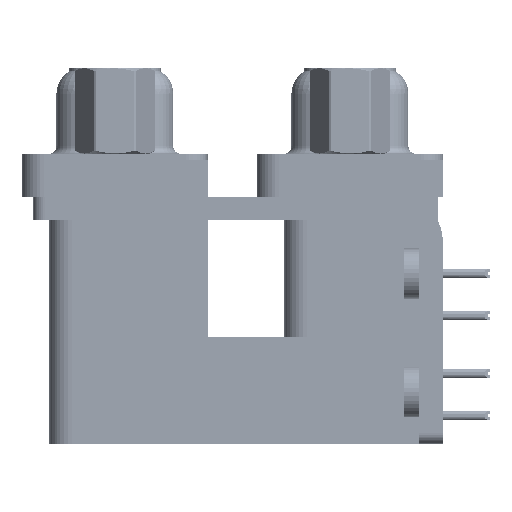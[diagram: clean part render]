
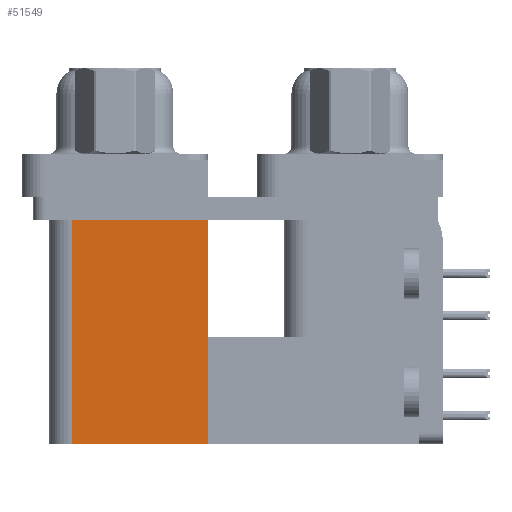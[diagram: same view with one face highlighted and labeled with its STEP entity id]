
A CAD part, left-side view. The second image highlights one B-rep face of the part: STEP entity #51549.
In plain terms, the highlighted planar face has unit normal (-1, 0, 0).
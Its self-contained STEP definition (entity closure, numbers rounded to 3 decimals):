
#265 = DIRECTION ( 'NONE',  ( 0., 0., 1. ) ) ;
#1208 = LINE ( 'NONE', #51632, #34394 ) ;
#1245 = VERTEX_POINT ( 'NONE', #5433 ) ;
#2728 = DIRECTION ( 'NONE',  ( 0., 1., 0. ) ) ;
#2841 = VECTOR ( 'NONE', #73169, 1000. ) ;
#5433 = CARTESIAN_POINT ( 'NONE',  ( 3.79, 18.8, -19.2 ) ) ;
#5642 = VERTEX_POINT ( 'NONE', #30023 ) ;
#8924 = LINE ( 'NONE', #34158, #12694 ) ;
#11295 = EDGE_CURVE ( 'NONE', #75592, #13830, #1208, .T. ) ;
#11579 = PLANE ( 'NONE',  #75513 ) ;
#11611 = ORIENTED_EDGE ( 'NONE', *, *, #14399, .F. ) ;
#12694 = VECTOR ( 'NONE', #2728, 1000. ) ;
#13830 = VERTEX_POINT ( 'NONE', #38008 ) ;
#14399 = EDGE_CURVE ( 'NONE', #75592, #1245, #8924, .T. ) ;
#16009 = CARTESIAN_POINT ( 'NONE',  ( 3.79, 9.6, -19.2 ) ) ;
#23456 = EDGE_CURVE ( 'NONE', #13830, #5642, #47955, .T. ) ;
#28058 = EDGE_CURVE ( 'NONE', #1245, #5642, #62277, .T. ) ;
#29595 = EDGE_LOOP ( 'NONE', ( #60127, #52604, #11611, #73415 ) ) ;
#30023 = CARTESIAN_POINT ( 'NONE',  ( 3.79, 18.8, -2.5 ) ) ;
#34158 = CARTESIAN_POINT ( 'NONE',  ( 3.79, 9.6, -19.2 ) ) ;
#34394 = VECTOR ( 'NONE', #64431, 1000. ) ;
#36811 = CARTESIAN_POINT ( 'NONE',  ( 3.79, 9.6, -19.2 ) ) ;
#38008 = CARTESIAN_POINT ( 'NONE',  ( 3.79, 9.6, -2.5 ) ) ;
#40959 = CARTESIAN_POINT ( 'NONE',  ( 3.79, 9.6, -2.5 ) ) ;
#43399 = DIRECTION ( 'NONE',  ( 0., 0., -1. ) ) ;
#47340 = VECTOR ( 'NONE', #265, 1000. ) ;
#47955 = LINE ( 'NONE', #40959, #2841 ) ;
#51549 = ADVANCED_FACE ( 'NONE', ( #68217 ), #11579, .F. ) ;
#51632 = CARTESIAN_POINT ( 'NONE',  ( 3.79, 9.6, -19.2 ) ) ;
#52604 = ORIENTED_EDGE ( 'NONE', *, *, #28058, .F. ) ;
#60127 = ORIENTED_EDGE ( 'NONE', *, *, #23456, .T. ) ;
#62277 = LINE ( 'NONE', #80488, #47340 ) ;
#64431 = DIRECTION ( 'NONE',  ( 0., 0., 1. ) ) ;
#68217 = FACE_OUTER_BOUND ( 'NONE', #29595, .T. ) ;
#73169 = DIRECTION ( 'NONE',  ( 0., 1., 0. ) ) ;
#73415 = ORIENTED_EDGE ( 'NONE', *, *, #11295, .T. ) ;
#75513 = AXIS2_PLACEMENT_3D ( 'NONE', #36811, #76036, #43399 ) ;
#75592 = VERTEX_POINT ( 'NONE', #16009 ) ;
#76036 = DIRECTION ( 'NONE',  ( 1., 0., 0. ) ) ;
#80488 = CARTESIAN_POINT ( 'NONE',  ( 3.79, 18.8, -19.2 ) ) ;
